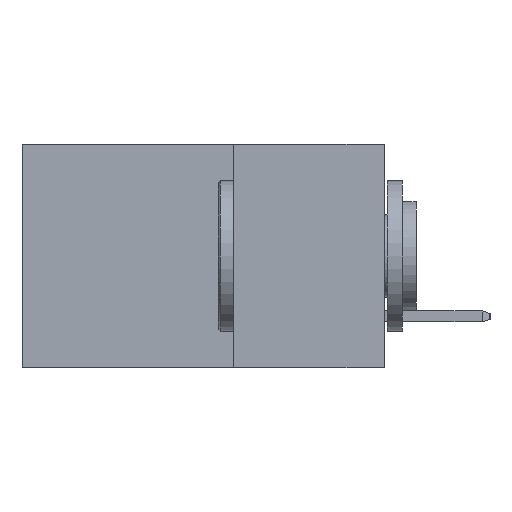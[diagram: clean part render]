
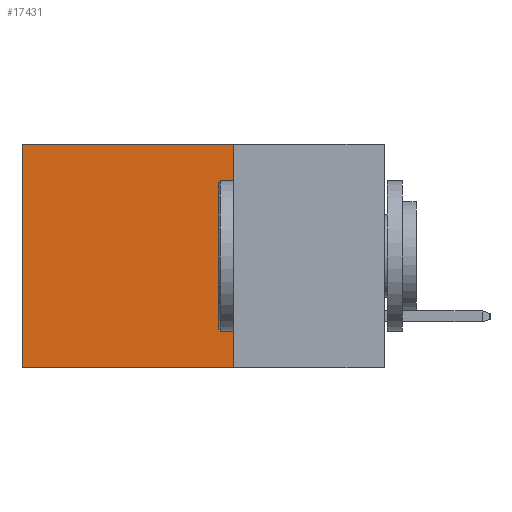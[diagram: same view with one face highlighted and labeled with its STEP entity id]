
A CAD part, left-side view. The second image highlights one B-rep face of the part: STEP entity #17431.
In plain terms, the highlighted planar face has unit normal (-1, 0, 0).
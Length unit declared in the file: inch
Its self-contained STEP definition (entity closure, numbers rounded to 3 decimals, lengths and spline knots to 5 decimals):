
#193 = EDGE_LOOP ( 'NONE', ( #17848, #10302, #9950, #18333 ) ) ;
#1283 = LINE ( 'NONE', #14828, #12980 ) ;
#1826 = CARTESIAN_POINT ( 'NONE',  ( 0.2615, 0.6, 0. ) ) ;
#2818 = LINE ( 'NONE', #7650, #6812 ) ;
#2937 = EDGE_CURVE ( 'NONE', #18077, #18739, #2818, .T. ) ;
#5338 = CARTESIAN_POINT ( 'NONE',  ( 0.2615, 0.25, -0.37 ) ) ;
#5483 = FACE_OUTER_BOUND ( 'NONE', #193, .T. ) ;
#5607 = DIRECTION ( 'NONE',  ( 0., 0., -1. ) ) ;
#5755 = LINE ( 'NONE', #5338, #13486 ) ;
#6422 = DIRECTION ( 'NONE',  ( 0., 1., 0. ) ) ;
#6423 = CARTESIAN_POINT ( 'NONE',  ( 0.2615, 0.6, -0.37 ) ) ;
#6531 = VERTEX_POINT ( 'NONE', #1826 ) ;
#6723 = EDGE_CURVE ( 'NONE', #19156, #18077, #5755, .T. ) ;
#6812 = VECTOR ( 'NONE', #6422, 39.37008 ) ;
#7349 = CARTESIAN_POINT ( 'NONE',  ( 0.2615, 0.25, -0.37 ) ) ;
#7650 = CARTESIAN_POINT ( 'NONE',  ( 0.2615, 0.25, -0.37 ) ) ;
#8389 = AXIS2_PLACEMENT_3D ( 'NONE', #7349, #18086, #8893 ) ;
#8893 = DIRECTION ( 'NONE',  ( 0., 0., -1. ) ) ;
#9950 = ORIENTED_EDGE ( 'NONE', *, *, #6723, .F. ) ;
#10302 = ORIENTED_EDGE ( 'NONE', *, *, #2937, .F. ) ;
#10624 = CARTESIAN_POINT ( 'NONE',  ( 0.2615, 0.6, -0.37 ) ) ;
#12980 = VECTOR ( 'NONE', #19256, 39.37008 ) ;
#13486 = VECTOR ( 'NONE', #5607, 39.37008 ) ;
#13698 = DIRECTION ( 'NONE',  ( 0., 0., -1. ) ) ;
#13884 = VECTOR ( 'NONE', #13698, 39.37008 ) ;
#14130 = CARTESIAN_POINT ( 'NONE',  ( 0.2615, 0.25, -0.37 ) ) ;
#14828 = CARTESIAN_POINT ( 'NONE',  ( 0.2615, 0.25, 0. ) ) ;
#15160 = CARTESIAN_POINT ( 'NONE',  ( 0.2615, 0.25, 0. ) ) ;
#15607 = EDGE_CURVE ( 'NONE', #19156, #6531, #1283, .T. ) ;
#16568 = PLANE ( 'NONE',  #8389 ) ;
#16824 = EDGE_CURVE ( 'NONE', #6531, #18739, #17958, .T. ) ;
#17431 = ADVANCED_FACE ( 'NONE', ( #5483 ), #16568, .F. ) ;
#17848 = ORIENTED_EDGE ( 'NONE', *, *, #16824, .T. ) ;
#17958 = LINE ( 'NONE', #10624, #13884 ) ;
#18077 = VERTEX_POINT ( 'NONE', #14130 ) ;
#18086 = DIRECTION ( 'NONE',  ( 1., 0., 0. ) ) ;
#18333 = ORIENTED_EDGE ( 'NONE', *, *, #15607, .T. ) ;
#18739 = VERTEX_POINT ( 'NONE', #6423 ) ;
#19156 = VERTEX_POINT ( 'NONE', #15160 ) ;
#19256 = DIRECTION ( 'NONE',  ( 0., 1., 0. ) ) ;
